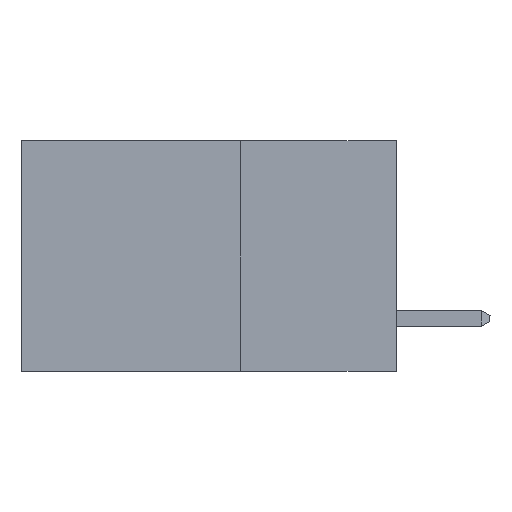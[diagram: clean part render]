
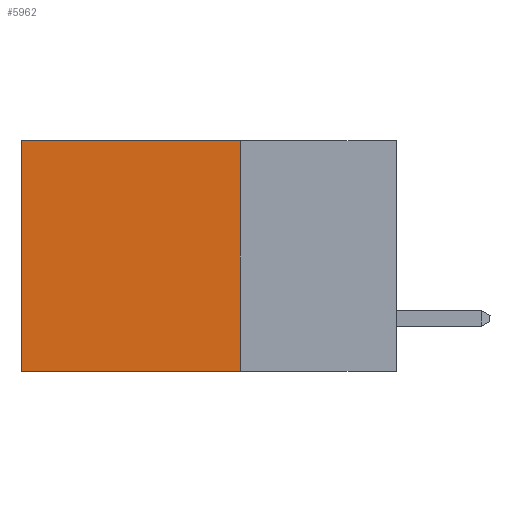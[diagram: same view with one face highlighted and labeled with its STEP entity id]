
A CAD part, left-side view. The second image highlights one B-rep face of the part: STEP entity #5962.
In plain terms, the highlighted planar face has unit normal (-1, 0, 0).
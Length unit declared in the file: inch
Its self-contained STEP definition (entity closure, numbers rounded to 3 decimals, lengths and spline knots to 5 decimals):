
#104 = CARTESIAN_POINT ( 'NONE',  ( 0.2615, 0.25, -0.37 ) ) ;
#236 = VERTEX_POINT ( 'NONE', #10943 ) ;
#1061 = EDGE_LOOP ( 'NONE', ( #9694, #4587, #12172, #4358 ) ) ;
#1254 = FACE_OUTER_BOUND ( 'NONE', #1061, .T. ) ;
#1418 = DIRECTION ( 'NONE',  ( 1., 0., 0. ) ) ;
#2125 = VECTOR ( 'NONE', #13192, 39.37008 ) ;
#2390 = LINE ( 'NONE', #13310, #10545 ) ;
#2501 = DIRECTION ( 'NONE',  ( 0., 0., -1. ) ) ;
#3190 = CARTESIAN_POINT ( 'NONE',  ( 0.2615, 0.6, 0. ) ) ;
#4284 = CARTESIAN_POINT ( 'NONE',  ( 0.2615, 0.25, 0. ) ) ;
#4358 = ORIENTED_EDGE ( 'NONE', *, *, #9446, .T. ) ;
#4470 = EDGE_CURVE ( 'NONE', #5672, #236, #12681, .T. ) ;
#4587 = ORIENTED_EDGE ( 'NONE', *, *, #12869, .F. ) ;
#4696 = CARTESIAN_POINT ( 'NONE',  ( 0.2615, 0.25, 0. ) ) ;
#5105 = EDGE_CURVE ( 'NONE', #10084, #9734, #8352, .T. ) ;
#5672 = VERTEX_POINT ( 'NONE', #4696 ) ;
#5962 = ADVANCED_FACE ( 'NONE', ( #1254 ), #12670, .F. ) ;
#6584 = DIRECTION ( 'NONE',  ( 0., 1., 0. ) ) ;
#7046 = VECTOR ( 'NONE', #6584, 39.37008 ) ;
#7148 = AXIS2_PLACEMENT_3D ( 'NONE', #7593, #1418, #2501 ) ;
#7593 = CARTESIAN_POINT ( 'NONE',  ( 0.2615, 0.25, -0.37 ) ) ;
#8073 = CARTESIAN_POINT ( 'NONE',  ( 0.2615, 0.6, -0.37 ) ) ;
#8352 = LINE ( 'NONE', #12021, #2125 ) ;
#9446 = EDGE_CURVE ( 'NONE', #5672, #10084, #11674, .T. ) ;
#9694 = ORIENTED_EDGE ( 'NONE', *, *, #5105, .T. ) ;
#9734 = VERTEX_POINT ( 'NONE', #8073 ) ;
#10084 = VERTEX_POINT ( 'NONE', #3190 ) ;
#10545 = VECTOR ( 'NONE', #14722, 39.37008 ) ;
#10943 = CARTESIAN_POINT ( 'NONE',  ( 0.2615, 0.25, -0.37 ) ) ;
#11674 = LINE ( 'NONE', #4284, #7046 ) ;
#12021 = CARTESIAN_POINT ( 'NONE',  ( 0.2615, 0.6, -0.37 ) ) ;
#12172 = ORIENTED_EDGE ( 'NONE', *, *, #4470, .F. ) ;
#12670 = PLANE ( 'NONE',  #7148 ) ;
#12681 = LINE ( 'NONE', #104, #15549 ) ;
#12869 = EDGE_CURVE ( 'NONE', #236, #9734, #2390, .T. ) ;
#13192 = DIRECTION ( 'NONE',  ( 0., 0., -1. ) ) ;
#13310 = CARTESIAN_POINT ( 'NONE',  ( 0.2615, 0.25, -0.37 ) ) ;
#14722 = DIRECTION ( 'NONE',  ( 0., 1., 0. ) ) ;
#15243 = DIRECTION ( 'NONE',  ( 0., 0., -1. ) ) ;
#15549 = VECTOR ( 'NONE', #15243, 39.37008 ) ;
